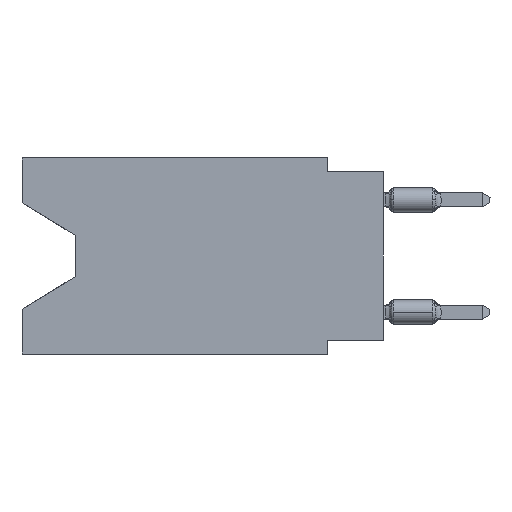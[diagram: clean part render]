
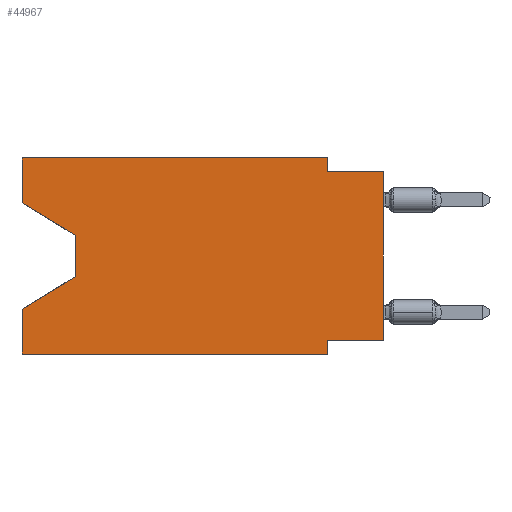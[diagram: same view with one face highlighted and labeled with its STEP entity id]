
A CAD part, left-side view. The second image highlights one B-rep face of the part: STEP entity #44967.
In plain terms, the highlighted planar face has unit normal (-1, 0, 0).
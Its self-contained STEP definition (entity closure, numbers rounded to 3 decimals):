
#445 = ORIENTED_EDGE ( 'NONE', *, *, #5132, .T. ) ;
#792 = CARTESIAN_POINT ( 'NONE',  ( 0., 2.54, -8.89 ) ) ;
#868 = DIRECTION ( 'NONE',  ( 0., 0., 1. ) ) ;
#940 = VECTOR ( 'NONE', #46475, 1000. ) ;
#1118 = CARTESIAN_POINT ( 'NONE',  ( 0., 16.383, 0. ) ) ;
#2305 = CARTESIAN_POINT ( 'NONE',  ( 0., 13.97, -3.505 ) ) ;
#2533 = ORIENTED_EDGE ( 'NONE', *, *, #15067, .T. ) ;
#2604 = ORIENTED_EDGE ( 'NONE', *, *, #8601, .F. ) ;
#2660 = DIRECTION ( 'NONE',  ( 0., -1., 0. ) ) ;
#3351 = FACE_OUTER_BOUND ( 'NONE', #34084, .T. ) ;
#4550 = VECTOR ( 'NONE', #22539, 1000. ) ;
#4815 = ORIENTED_EDGE ( 'NONE', *, *, #18453, .F. ) ;
#5132 = EDGE_CURVE ( 'NONE', #43401, #39216, #45623, .T. ) ;
#5662 = CARTESIAN_POINT ( 'NONE',  ( 0., 13.97, -5.385 ) ) ;
#5829 = DIRECTION ( 'NONE',  ( 0., 0., 1. ) ) ;
#6143 = AXIS2_PLACEMENT_3D ( 'NONE', #10999, #11715, #34083 ) ;
#6179 = CARTESIAN_POINT ( 'NONE',  ( 0., 16.383, -2.038 ) ) ;
#6832 = VERTEX_POINT ( 'NONE', #34080 ) ;
#8142 = VECTOR ( 'NONE', #23281, 1000. ) ;
#8601 = EDGE_CURVE ( 'NONE', #14953, #34081, #38231, .T. ) ;
#8715 = ORIENTED_EDGE ( 'NONE', *, *, #17843, .T. ) ;
#9784 = CARTESIAN_POINT ( 'NONE',  ( 0., 16.383, 0. ) ) ;
#9989 = VERTEX_POINT ( 'NONE', #34287 ) ;
#10331 = CARTESIAN_POINT ( 'NONE',  ( 0., 2.54, -8.89 ) ) ;
#10541 = VERTEX_POINT ( 'NONE', #5662 ) ;
#10999 = CARTESIAN_POINT ( 'NONE',  ( 0., 16.383, 0. ) ) ;
#11094 = CARTESIAN_POINT ( 'NONE',  ( 0., 2.54, 0. ) ) ;
#11101 = VECTOR ( 'NONE', #5829, 1000. ) ;
#11360 = LINE ( 'NONE', #41639, #4550 ) ;
#11715 = DIRECTION ( 'NONE',  ( 1., 0., 0. ) ) ;
#12255 = VECTOR ( 'NONE', #2660, 1000. ) ;
#13410 = EDGE_CURVE ( 'NONE', #27009, #42590, #34843, .T. ) ;
#13476 = ORIENTED_EDGE ( 'NONE', *, *, #39176, .F. ) ;
#14123 = VERTEX_POINT ( 'NONE', #19298 ) ;
#14953 = VERTEX_POINT ( 'NONE', #48327 ) ;
#15067 = EDGE_CURVE ( 'NONE', #21203, #10541, #46516, .T. ) ;
#15829 = CARTESIAN_POINT ( 'NONE',  ( 0., 16.383, -8.89 ) ) ;
#15892 = DIRECTION ( 'NONE',  ( 0., -1., 0. ) ) ;
#16724 = VECTOR ( 'NONE', #15892, 1000. ) ;
#17843 = EDGE_CURVE ( 'NONE', #38595, #34081, #46867, .T. ) ;
#18453 = EDGE_CURVE ( 'NONE', #43401, #9989, #40043, .T. ) ;
#19237 = ORIENTED_EDGE ( 'NONE', *, *, #26497, .F. ) ;
#19298 = CARTESIAN_POINT ( 'NONE',  ( 0., 2.54, 0. ) ) ;
#21203 = VERTEX_POINT ( 'NONE', #2305 ) ;
#22223 = CARTESIAN_POINT ( 'NONE',  ( 0., 13.97, -5.385 ) ) ;
#22539 = DIRECTION ( 'NONE',  ( 0., -0.855, -0.519 ) ) ;
#22733 = LINE ( 'NONE', #11094, #30781 ) ;
#23102 = EDGE_CURVE ( 'NONE', #10541, #9989, #36866, .T. ) ;
#23281 = DIRECTION ( 'NONE',  ( 0., -1., 0. ) ) ;
#23366 = CARTESIAN_POINT ( 'NONE',  ( 0., 0., -8.255 ) ) ;
#23739 = DIRECTION ( 'NONE',  ( 0., 0., 1. ) ) ;
#24096 = CARTESIAN_POINT ( 'NONE',  ( 0., 0., -0.635 ) ) ;
#26497 = EDGE_CURVE ( 'NONE', #6832, #39216, #38735, .T. ) ;
#26679 = ORIENTED_EDGE ( 'NONE', *, *, #33058, .F. ) ;
#26851 = VECTOR ( 'NONE', #868, 1000. ) ;
#27009 = VERTEX_POINT ( 'NONE', #6179 ) ;
#27104 = EDGE_CURVE ( 'NONE', #14123, #14953, #22733, .T. ) ;
#28328 = ORIENTED_EDGE ( 'NONE', *, *, #47299, .T. ) ;
#29472 = ORIENTED_EDGE ( 'NONE', *, *, #27104, .F. ) ;
#30747 = VECTOR ( 'NONE', #41329, 1000. ) ;
#30752 = CARTESIAN_POINT ( 'NONE',  ( 0., 16.383, 0. ) ) ;
#30781 = VECTOR ( 'NONE', #34173, 1000. ) ;
#32173 = CARTESIAN_POINT ( 'NONE',  ( 0., 0., 0. ) ) ;
#33058 = EDGE_CURVE ( 'NONE', #38595, #6832, #42254, .T. ) ;
#33907 = CARTESIAN_POINT ( 'NONE',  ( 0., 0., -0.635 ) ) ;
#34080 = CARTESIAN_POINT ( 'NONE',  ( 0., 2.54, -8.255 ) ) ;
#34081 = VERTEX_POINT ( 'NONE', #33907 ) ;
#34083 = DIRECTION ( 'NONE',  ( 0., 0., -1. ) ) ;
#34084 = EDGE_LOOP ( 'NONE', ( #28328, #2533, #36123, #4815, #445, #19237, #26679, #8715, #2604, #29472, #13476, #38160 ) ) ;
#34173 = DIRECTION ( 'NONE',  ( 0., 0., -1. ) ) ;
#34287 = CARTESIAN_POINT ( 'NONE',  ( 0., 16.383, -6.852 ) ) ;
#34843 = LINE ( 'NONE', #1118, #26851 ) ;
#36123 = ORIENTED_EDGE ( 'NONE', *, *, #23102, .T. ) ;
#36866 = LINE ( 'NONE', #22223, #30747 ) ;
#36872 = LINE ( 'NONE', #44339, #12255 ) ;
#37615 = CARTESIAN_POINT ( 'NONE',  ( 0., 16.383, -8.89 ) ) ;
#38160 = ORIENTED_EDGE ( 'NONE', *, *, #13410, .F. ) ;
#38231 = LINE ( 'NONE', #24096, #16724 ) ;
#38534 = CARTESIAN_POINT ( 'NONE',  ( 0., 13.97, -3.505 ) ) ;
#38595 = VERTEX_POINT ( 'NONE', #43423 ) ;
#38735 = LINE ( 'NONE', #792, #44287 ) ;
#39176 = EDGE_CURVE ( 'NONE', #42590, #14123, #36872, .T. ) ;
#39216 = VERTEX_POINT ( 'NONE', #10331 ) ;
#40043 = LINE ( 'NONE', #9784, #11101 ) ;
#40720 = DIRECTION ( 'NONE',  ( 0., 0., -1. ) ) ;
#41329 = DIRECTION ( 'NONE',  ( 0., 0.855, -0.519 ) ) ;
#41530 = PLANE ( 'NONE',  #6143 ) ;
#41639 = CARTESIAN_POINT ( 'NONE',  ( 0., 16.383, -2.038 ) ) ;
#42254 = LINE ( 'NONE', #23366, #940 ) ;
#42590 = VERTEX_POINT ( 'NONE', #30752 ) ;
#43401 = VERTEX_POINT ( 'NONE', #37615 ) ;
#43423 = CARTESIAN_POINT ( 'NONE',  ( 0., 0., -8.255 ) ) ;
#44287 = VECTOR ( 'NONE', #40720, 1000. ) ;
#44339 = CARTESIAN_POINT ( 'NONE',  ( 0., 16.383, 0. ) ) ;
#44400 = VECTOR ( 'NONE', #23739, 1000. ) ;
#44967 = ADVANCED_FACE ( 'NONE', ( #3351 ), #41530, .F. ) ;
#45623 = LINE ( 'NONE', #15829, #8142 ) ;
#46267 = DIRECTION ( 'NONE',  ( 0., 0., -1. ) ) ;
#46372 = VECTOR ( 'NONE', #46267, 1000. ) ;
#46475 = DIRECTION ( 'NONE',  ( 0., 1., 0. ) ) ;
#46516 = LINE ( 'NONE', #38534, #46372 ) ;
#46867 = LINE ( 'NONE', #32173, #44400 ) ;
#47299 = EDGE_CURVE ( 'NONE', #27009, #21203, #11360, .T. ) ;
#48327 = CARTESIAN_POINT ( 'NONE',  ( 0., 2.54, -0.635 ) ) ;
